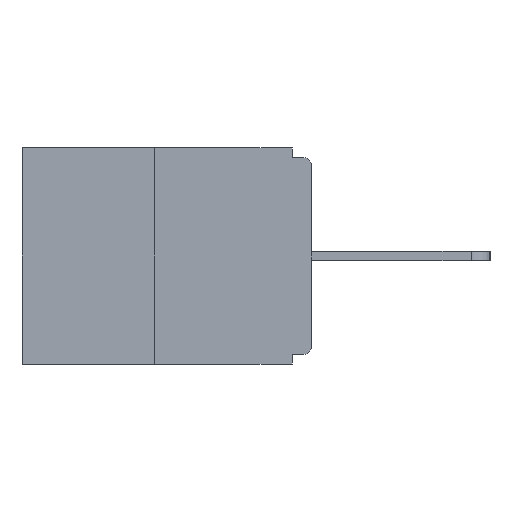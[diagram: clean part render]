
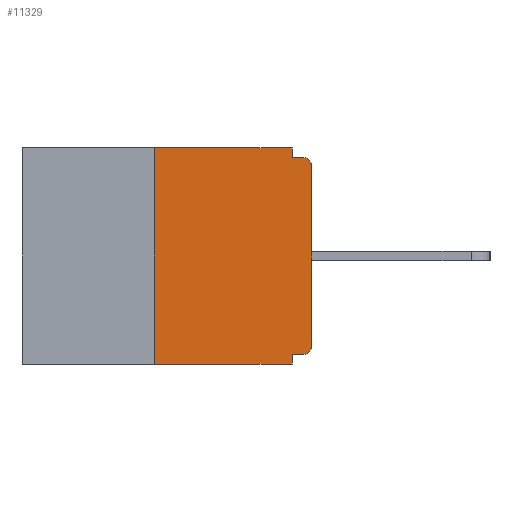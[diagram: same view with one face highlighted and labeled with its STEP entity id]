
A CAD part, left-side view. The second image highlights one B-rep face of the part: STEP entity #11329.
In plain terms, the highlighted planar face has unit normal (-1, 0, 0).
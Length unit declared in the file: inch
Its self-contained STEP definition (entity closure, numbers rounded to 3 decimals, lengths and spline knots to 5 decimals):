
#476 = ORIENTED_EDGE ( 'NONE', *, *, #21503, .F. ) ;
#1227 = EDGE_LOOP ( 'NONE', ( #21696, #14463, #13786, #14892, #15725, #18752, #14270, #7427, #476, #8235 ) ) ;
#1860 = VERTEX_POINT ( 'NONE', #5923 ) ;
#2049 = CARTESIAN_POINT ( 'NONE',  ( 0., 0.031, -0.343 ) ) ;
#2182 = CARTESIAN_POINT ( 'NONE',  ( 0., 0.015, -0.03 ) ) ;
#2491 = CARTESIAN_POINT ( 'NONE',  ( 0., 0.015, -0.328 ) ) ;
#2640 = FACE_OUTER_BOUND ( 'NONE', #1227, .T. ) ;
#2781 = CARTESIAN_POINT ( 'NONE',  ( 0., 0.031, -0.328 ) ) ;
#2982 = LINE ( 'NONE', #21952, #8087 ) ;
#3526 = DIRECTION ( 'NONE',  ( 0., 0., -1. ) ) ;
#3660 = LINE ( 'NONE', #13698, #12321 ) ;
#3797 = VERTEX_POINT ( 'NONE', #5974 ) ;
#4181 = CARTESIAN_POINT ( 'NONE',  ( 0., 0.25, 0. ) ) ;
#4580 = EDGE_CURVE ( 'NONE', #15544, #21056, #6773, .T. ) ;
#5085 = DIRECTION ( 'NONE',  ( 0., 0., 1. ) ) ;
#5628 = EDGE_CURVE ( 'NONE', #7833, #16449, #14305, .T. ) ;
#5665 = EDGE_CURVE ( 'NONE', #15544, #7833, #19454, .T. ) ;
#5710 = DIRECTION ( 'NONE',  ( 0., 1., 0. ) ) ;
#5732 = CARTESIAN_POINT ( 'NONE',  ( 0., 0., -0.313 ) ) ;
#5848 = LINE ( 'NONE', #16326, #21623 ) ;
#5923 = CARTESIAN_POINT ( 'NONE',  ( 0., 0.25, -0.343 ) ) ;
#5974 = CARTESIAN_POINT ( 'NONE',  ( 0., 0., -0.03 ) ) ;
#6189 = PLANE ( 'NONE',  #18356 ) ;
#6505 = VERTEX_POINT ( 'NONE', #4181 ) ;
#6773 = CIRCLE ( 'NONE', #19959, 0.015 ) ;
#7103 = CARTESIAN_POINT ( 'NONE',  ( 0., 0.015, -0.313 ) ) ;
#7297 = DIRECTION ( 'NONE',  ( -1., 0., 0. ) ) ;
#7427 = ORIENTED_EDGE ( 'NONE', *, *, #13714, .T. ) ;
#7833 = VERTEX_POINT ( 'NONE', #2781 ) ;
#8087 = VECTOR ( 'NONE', #5085, 39.37008 ) ;
#8235 = ORIENTED_EDGE ( 'NONE', *, *, #13361, .F. ) ;
#8346 = DIRECTION ( 'NONE',  ( 0., -1., 0. ) ) ;
#8563 = CARTESIAN_POINT ( 'NONE',  ( 0., 0.015, -0.015 ) ) ;
#8780 = DIRECTION ( 'NONE',  ( 0., 0., -1. ) ) ;
#8808 = VERTEX_POINT ( 'NONE', #13185 ) ;
#9054 = CARTESIAN_POINT ( 'NONE',  ( 0., 0., -0.328 ) ) ;
#9573 = CARTESIAN_POINT ( 'NONE',  ( 0., 0., -0.015 ) ) ;
#10202 = CIRCLE ( 'NONE', #14842, 0.015 ) ;
#10732 = CARTESIAN_POINT ( 'NONE',  ( 0., 0.031, -0.343 ) ) ;
#11073 = VECTOR ( 'NONE', #5710, 39.37008 ) ;
#11300 = EDGE_CURVE ( 'NONE', #1860, #16449, #11431, .T. ) ;
#11329 = ADVANCED_FACE ( 'NONE', ( #2640 ), #6189, .F. ) ;
#11431 = LINE ( 'NONE', #14558, #18711 ) ;
#12321 = VECTOR ( 'NONE', #13914, 39.37008 ) ;
#13185 = CARTESIAN_POINT ( 'NONE',  ( 0., 0.031, 0. ) ) ;
#13361 = EDGE_CURVE ( 'NONE', #8808, #13582, #3660, .T. ) ;
#13366 = VECTOR ( 'NONE', #21653, 39.37008 ) ;
#13582 = VERTEX_POINT ( 'NONE', #16570 ) ;
#13698 = CARTESIAN_POINT ( 'NONE',  ( 0., 0.031, 0. ) ) ;
#13714 = EDGE_CURVE ( 'NONE', #3797, #18671, #10202, .T. ) ;
#13786 = ORIENTED_EDGE ( 'NONE', *, *, #11300, .T. ) ;
#13903 = EDGE_CURVE ( 'NONE', #21056, #3797, #5848, .T. ) ;
#13914 = DIRECTION ( 'NONE',  ( 0., 0., -1. ) ) ;
#13917 = DIRECTION ( 'NONE',  ( -1., 0., 0. ) ) ;
#13969 = VECTOR ( 'NONE', #8346, 39.37008 ) ;
#14270 = ORIENTED_EDGE ( 'NONE', *, *, #13903, .T. ) ;
#14305 = LINE ( 'NONE', #10732, #16048 ) ;
#14328 = DIRECTION ( 'NONE',  ( 0., 0., 1. ) ) ;
#14463 = ORIENTED_EDGE ( 'NONE', *, *, #14851, .F. ) ;
#14558 = CARTESIAN_POINT ( 'NONE',  ( 0., 0.46, -0.343 ) ) ;
#14842 = AXIS2_PLACEMENT_3D ( 'NONE', #2182, #7297, #3526 ) ;
#14851 = EDGE_CURVE ( 'NONE', #1860, #6505, #2982, .T. ) ;
#14892 = ORIENTED_EDGE ( 'NONE', *, *, #5628, .F. ) ;
#15260 = CARTESIAN_POINT ( 'NONE',  ( 0., 0.46, 0. ) ) ;
#15544 = VERTEX_POINT ( 'NONE', #2491 ) ;
#15725 = ORIENTED_EDGE ( 'NONE', *, *, #5665, .F. ) ;
#16048 = VECTOR ( 'NONE', #17541, 39.37008 ) ;
#16326 = CARTESIAN_POINT ( 'NONE',  ( 0., 0., 0. ) ) ;
#16445 = CARTESIAN_POINT ( 'NONE',  ( 0., 0.46, 0. ) ) ;
#16449 = VERTEX_POINT ( 'NONE', #2049 ) ;
#16570 = CARTESIAN_POINT ( 'NONE',  ( 0., 0.031, -0.015 ) ) ;
#17313 = EDGE_CURVE ( 'NONE', #6505, #8808, #20201, .T. ) ;
#17541 = DIRECTION ( 'NONE',  ( 0., 0., -1. ) ) ;
#18356 = AXIS2_PLACEMENT_3D ( 'NONE', #16445, #21277, #21493 ) ;
#18671 = VERTEX_POINT ( 'NONE', #8563 ) ;
#18711 = VECTOR ( 'NONE', #21381, 39.37008 ) ;
#18752 = ORIENTED_EDGE ( 'NONE', *, *, #4580, .T. ) ;
#19454 = LINE ( 'NONE', #9054, #11073 ) ;
#19959 = AXIS2_PLACEMENT_3D ( 'NONE', #7103, #13917, #8780 ) ;
#20201 = LINE ( 'NONE', #15260, #13969 ) ;
#21056 = VERTEX_POINT ( 'NONE', #5732 ) ;
#21277 = DIRECTION ( 'NONE',  ( 1., 0., 0. ) ) ;
#21320 = LINE ( 'NONE', #9573, #13366 ) ;
#21381 = DIRECTION ( 'NONE',  ( 0., -1., 0. ) ) ;
#21493 = DIRECTION ( 'NONE',  ( 0., 0., -1. ) ) ;
#21503 = EDGE_CURVE ( 'NONE', #13582, #18671, #21320, .T. ) ;
#21623 = VECTOR ( 'NONE', #14328, 39.37008 ) ;
#21653 = DIRECTION ( 'NONE',  ( 0., -1., 0. ) ) ;
#21696 = ORIENTED_EDGE ( 'NONE', *, *, #17313, .F. ) ;
#21952 = CARTESIAN_POINT ( 'NONE',  ( 0., 0.25, 0. ) ) ;
